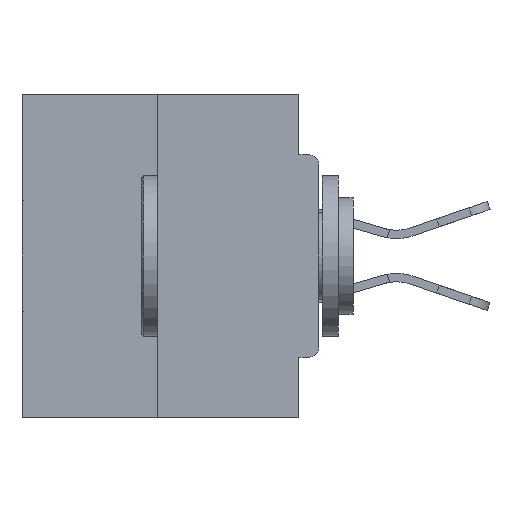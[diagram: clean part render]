
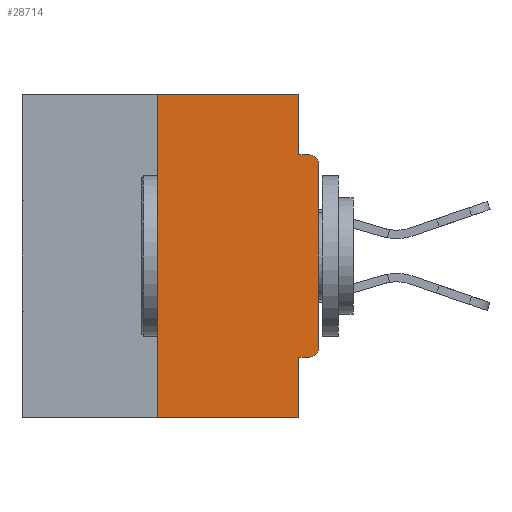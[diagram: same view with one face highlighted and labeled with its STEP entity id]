
A CAD part, left-side view. The second image highlights one B-rep face of the part: STEP entity #28714.
In plain terms, the highlighted planar face has unit normal (-1, 0, 0).
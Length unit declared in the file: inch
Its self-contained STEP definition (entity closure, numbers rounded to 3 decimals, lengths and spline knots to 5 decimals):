
#431 = CARTESIAN_POINT ( 'NONE',  ( 0., 0.015, -0.3915 ) ) ;
#654 = AXIS2_PLACEMENT_3D ( 'NONE', #431, #3030, #9766 ) ;
#1379 = ORIENTED_EDGE ( 'NONE', *, *, #31229, .F. ) ;
#2042 = VERTEX_POINT ( 'NONE', #25633 ) ;
#2182 = CARTESIAN_POINT ( 'NONE',  ( 0., 0.015, -0.1085 ) ) ;
#2785 = DIRECTION ( 'NONE',  ( 0., 0., 1. ) ) ;
#3023 = VECTOR ( 'NONE', #2785, 39.37008 ) ;
#3030 = DIRECTION ( 'NONE',  ( -1., 0., 0. ) ) ;
#3053 = CARTESIAN_POINT ( 'NONE',  ( 0., 0., 0. ) ) ;
#3198 = DIRECTION ( 'NONE',  ( 0., 0., -1. ) ) ;
#3241 = CARTESIAN_POINT ( 'NONE',  ( 0., 0.46, 0. ) ) ;
#3581 = CARTESIAN_POINT ( 'NONE',  ( 0., 0.015, -0.4065 ) ) ;
#3769 = ORIENTED_EDGE ( 'NONE', *, *, #29473, .T. ) ;
#4004 = LINE ( 'NONE', #3053, #3023 ) ;
#4624 = VERTEX_POINT ( 'NONE', #21901 ) ;
#4985 = DIRECTION ( 'NONE',  ( 0., 0., 1. ) ) ;
#5272 = ORIENTED_EDGE ( 'NONE', *, *, #19864, .T. ) ;
#5304 = DIRECTION ( 'NONE',  ( 0., -1., 0. ) ) ;
#5367 = DIRECTION ( 'NONE',  ( -1., 0., 0. ) ) ;
#6309 = CARTESIAN_POINT ( 'NONE',  ( 0., 0.031, 0. ) ) ;
#6670 = VECTOR ( 'NONE', #34776, 39.37008 ) ;
#6778 = ORIENTED_EDGE ( 'NONE', *, *, #11700, .T. ) ;
#7348 = CARTESIAN_POINT ( 'NONE',  ( 0., 0.25, -0.5 ) ) ;
#7384 = EDGE_CURVE ( 'NONE', #9359, #38622, #9148, .T. ) ;
#9148 = LINE ( 'NONE', #37862, #27733 ) ;
#9269 = CIRCLE ( 'NONE', #654, 0.015 ) ;
#9359 = VERTEX_POINT ( 'NONE', #3581 ) ;
#9766 = DIRECTION ( 'NONE',  ( 0., 0., -1. ) ) ;
#9914 = EDGE_CURVE ( 'NONE', #39365, #2042, #4004, .T. ) ;
#11070 = EDGE_LOOP ( 'NONE', ( #22691, #31859, #6778, #37414, #17210, #3769, #30800, #5272, #1379, #37299 ) ) ;
#11332 = EDGE_CURVE ( 'NONE', #38591, #15300, #30783, .T. ) ;
#11700 = EDGE_CURVE ( 'NONE', #38591, #4624, #27348, .T. ) ;
#12820 = CARTESIAN_POINT ( 'NONE',  ( 0., 0.46, 0. ) ) ;
#12924 = EDGE_CURVE ( 'NONE', #32653, #36404, #25755, .T. ) ;
#13589 = VECTOR ( 'NONE', #5304, 39.37008 ) ;
#14045 = LINE ( 'NONE', #20893, #13589 ) ;
#14781 = LINE ( 'NONE', #20035, #25062 ) ;
#14782 = CARTESIAN_POINT ( 'NONE',  ( 0., 0.031, 0. ) ) ;
#15203 = EDGE_CURVE ( 'NONE', #15300, #32653, #30854, .T. ) ;
#15300 = VERTEX_POINT ( 'NONE', #29211 ) ;
#17210 = ORIENTED_EDGE ( 'NONE', *, *, #7384, .F. ) ;
#18054 = VECTOR ( 'NONE', #19605, 39.37008 ) ;
#19605 = DIRECTION ( 'NONE',  ( 0., -1., 0. ) ) ;
#19864 = EDGE_CURVE ( 'NONE', #2042, #39995, #20235, .T. ) ;
#20035 = CARTESIAN_POINT ( 'NONE',  ( 0., 0.031, -0.5 ) ) ;
#20235 = CIRCLE ( 'NONE', #35532, 0.015 ) ;
#20855 = CARTESIAN_POINT ( 'NONE',  ( 0., 0.25, 0. ) ) ;
#20893 = CARTESIAN_POINT ( 'NONE',  ( 0., 0., -0.0935 ) ) ;
#21716 = DIRECTION ( 'NONE',  ( 0., -1., 0. ) ) ;
#21901 = CARTESIAN_POINT ( 'NONE',  ( 0., 0.031, -0.5 ) ) ;
#22691 = ORIENTED_EDGE ( 'NONE', *, *, #15203, .F. ) ;
#25062 = VECTOR ( 'NONE', #29162, 39.37008 ) ;
#25633 = CARTESIAN_POINT ( 'NONE',  ( 0., 0., -0.1085 ) ) ;
#25755 = LINE ( 'NONE', #6309, #6670 ) ;
#27019 = CARTESIAN_POINT ( 'NONE',  ( 0., 0.031, -0.0935 ) ) ;
#27245 = DIRECTION ( 'NONE',  ( 0., 0., -1. ) ) ;
#27348 = LINE ( 'NONE', #28881, #18054 ) ;
#27733 = VECTOR ( 'NONE', #31753, 39.37008 ) ;
#28059 = EDGE_CURVE ( 'NONE', #38622, #4624, #14781, .T. ) ;
#28259 = PLANE ( 'NONE',  #35904 ) ;
#28714 = ADVANCED_FACE ( 'NONE', ( #33212 ), #28259, .F. ) ;
#28881 = CARTESIAN_POINT ( 'NONE',  ( 0., 0.46, -0.5 ) ) ;
#29162 = DIRECTION ( 'NONE',  ( 0., 0., -1. ) ) ;
#29211 = CARTESIAN_POINT ( 'NONE',  ( 0., 0.25, 0. ) ) ;
#29473 = EDGE_CURVE ( 'NONE', #9359, #39365, #9269, .T. ) ;
#30783 = LINE ( 'NONE', #20855, #40011 ) ;
#30800 = ORIENTED_EDGE ( 'NONE', *, *, #9914, .T. ) ;
#30854 = LINE ( 'NONE', #3241, #31316 ) ;
#31229 = EDGE_CURVE ( 'NONE', #36404, #39995, #14045, .T. ) ;
#31316 = VECTOR ( 'NONE', #21716, 39.37008 ) ;
#31381 = DIRECTION ( 'NONE',  ( 1., 0., 0. ) ) ;
#31753 = DIRECTION ( 'NONE',  ( 0., 1., 0. ) ) ;
#31859 = ORIENTED_EDGE ( 'NONE', *, *, #11332, .F. ) ;
#32653 = VERTEX_POINT ( 'NONE', #14782 ) ;
#33212 = FACE_OUTER_BOUND ( 'NONE', #11070, .T. ) ;
#34776 = DIRECTION ( 'NONE',  ( 0., 0., -1. ) ) ;
#35532 = AXIS2_PLACEMENT_3D ( 'NONE', #2182, #5367, #27245 ) ;
#35904 = AXIS2_PLACEMENT_3D ( 'NONE', #12820, #31381, #3198 ) ;
#35959 = CARTESIAN_POINT ( 'NONE',  ( 0., 0., -0.3915 ) ) ;
#36404 = VERTEX_POINT ( 'NONE', #27019 ) ;
#36648 = CARTESIAN_POINT ( 'NONE',  ( 0., 0.015, -0.0935 ) ) ;
#37299 = ORIENTED_EDGE ( 'NONE', *, *, #12924, .F. ) ;
#37414 = ORIENTED_EDGE ( 'NONE', *, *, #28059, .F. ) ;
#37862 = CARTESIAN_POINT ( 'NONE',  ( 0., 0., -0.4065 ) ) ;
#38562 = CARTESIAN_POINT ( 'NONE',  ( 0., 0.031, -0.4065 ) ) ;
#38591 = VERTEX_POINT ( 'NONE', #7348 ) ;
#38622 = VERTEX_POINT ( 'NONE', #38562 ) ;
#39365 = VERTEX_POINT ( 'NONE', #35959 ) ;
#39995 = VERTEX_POINT ( 'NONE', #36648 ) ;
#40011 = VECTOR ( 'NONE', #4985, 39.37008 ) ;
